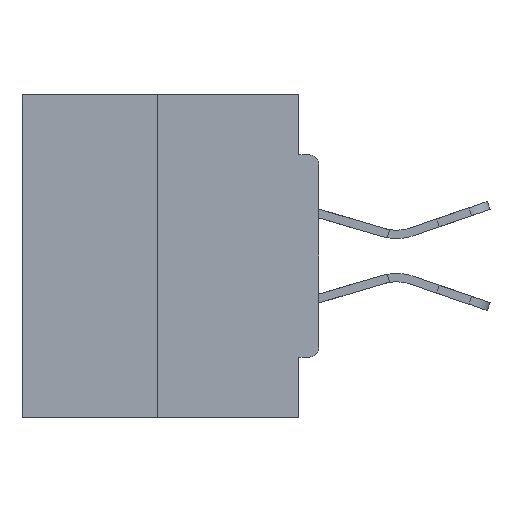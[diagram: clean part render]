
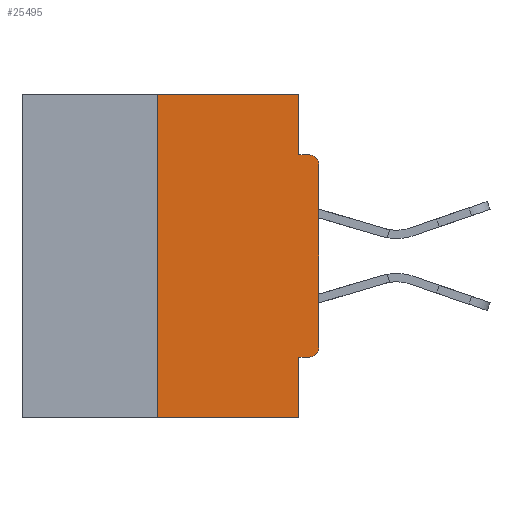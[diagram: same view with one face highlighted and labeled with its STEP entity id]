
A CAD part, left-side view. The second image highlights one B-rep face of the part: STEP entity #25495.
In plain terms, the highlighted planar face has unit normal (-1, 0, 0).
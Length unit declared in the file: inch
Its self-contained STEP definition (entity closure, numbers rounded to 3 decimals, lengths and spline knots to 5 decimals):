
#84 = ORIENTED_EDGE ( 'NONE', *, *, #33081, .F. ) ;
#152 = LINE ( 'NONE', #28186, #579 ) ;
#579 = VECTOR ( 'NONE', #2247, 39.37008 ) ;
#937 = DIRECTION ( 'NONE',  ( 1., 0., 0. ) ) ;
#1289 = VERTEX_POINT ( 'NONE', #6675 ) ;
#1444 = EDGE_CURVE ( 'NONE', #12754, #9517, #26013, .T. ) ;
#2247 = DIRECTION ( 'NONE',  ( 0., -1., 0. ) ) ;
#2290 = DIRECTION ( 'NONE',  ( 0., 0., 1. ) ) ;
#2374 = AXIS2_PLACEMENT_3D ( 'NONE', #28619, #2547, #28486 ) ;
#2547 = DIRECTION ( 'NONE',  ( -1., 0., 0. ) ) ;
#2644 = LINE ( 'NONE', #3035, #33446 ) ;
#3035 = CARTESIAN_POINT ( 'NONE',  ( 0., 0.46, 0. ) ) ;
#3228 = VERTEX_POINT ( 'NONE', #19448 ) ;
#3756 = PLANE ( 'NONE',  #8763 ) ;
#3840 = DIRECTION ( 'NONE',  ( 0., 0., -1. ) ) ;
#4269 = ORIENTED_EDGE ( 'NONE', *, *, #28178, .T. ) ;
#4535 = CARTESIAN_POINT ( 'NONE',  ( 0., 0.031, 0. ) ) ;
#5075 = AXIS2_PLACEMENT_3D ( 'NONE', #9763, #35532, #3840 ) ;
#5079 = EDGE_CURVE ( 'NONE', #5355, #14339, #24553, .T. ) ;
#5355 = VERTEX_POINT ( 'NONE', #33275 ) ;
#6125 = DIRECTION ( 'NONE',  ( 0., 0., -1. ) ) ;
#6675 = CARTESIAN_POINT ( 'NONE',  ( 0., 0.25, 0. ) ) ;
#7234 = EDGE_CURVE ( 'NONE', #9517, #19406, #33463, .T. ) ;
#7672 = EDGE_CURVE ( 'NONE', #36453, #3228, #17174, .T. ) ;
#8690 = CARTESIAN_POINT ( 'NONE',  ( 0., 0., -0.1085 ) ) ;
#8763 = AXIS2_PLACEMENT_3D ( 'NONE', #17320, #937, #26868 ) ;
#9124 = CARTESIAN_POINT ( 'NONE',  ( 0., 0., -0.0935 ) ) ;
#9208 = DIRECTION ( 'NONE',  ( 0., -1., 0. ) ) ;
#9387 = CARTESIAN_POINT ( 'NONE',  ( 0., 0.25, -0.5 ) ) ;
#9517 = VERTEX_POINT ( 'NONE', #10937 ) ;
#9763 = CARTESIAN_POINT ( 'NONE',  ( 0., 0.015, -0.3915 ) ) ;
#10514 = VERTEX_POINT ( 'NONE', #8690 ) ;
#10799 = VECTOR ( 'NONE', #27660, 39.37008 ) ;
#10937 = CARTESIAN_POINT ( 'NONE',  ( 0., 0.031, -0.0935 ) ) ;
#12011 = DIRECTION ( 'NONE',  ( 0., -1., 0. ) ) ;
#12162 = CARTESIAN_POINT ( 'NONE',  ( 0., 0.031, -0.5 ) ) ;
#12621 = LINE ( 'NONE', #24603, #10799 ) ;
#12754 = VERTEX_POINT ( 'NONE', #4535 ) ;
#13917 = CARTESIAN_POINT ( 'NONE',  ( 0., 0., 0. ) ) ;
#14274 = VECTOR ( 'NONE', #15642, 39.37008 ) ;
#14317 = VECTOR ( 'NONE', #25302, 39.37008 ) ;
#14339 = VERTEX_POINT ( 'NONE', #31032 ) ;
#14480 = ORIENTED_EDGE ( 'NONE', *, *, #7234, .F. ) ;
#14607 = ORIENTED_EDGE ( 'NONE', *, *, #34176, .T. ) ;
#15642 = DIRECTION ( 'NONE',  ( 0., 0., -1. ) ) ;
#15994 = CARTESIAN_POINT ( 'NONE',  ( 0., 0.015, -0.4065 ) ) ;
#16292 = ORIENTED_EDGE ( 'NONE', *, *, #23053, .F. ) ;
#17012 = ORIENTED_EDGE ( 'NONE', *, *, #22709, .F. ) ;
#17174 = CIRCLE ( 'NONE', #5075, 0.015 ) ;
#17320 = CARTESIAN_POINT ( 'NONE',  ( 0., 0.46, 0. ) ) ;
#18474 = EDGE_CURVE ( 'NONE', #25018, #14339, #152, .T. ) ;
#19049 = CIRCLE ( 'NONE', #2374, 0.015 ) ;
#19406 = VERTEX_POINT ( 'NONE', #34623 ) ;
#19448 = CARTESIAN_POINT ( 'NONE',  ( 0., 0., -0.3915 ) ) ;
#19876 = CARTESIAN_POINT ( 'NONE',  ( 0., 0.25, 0. ) ) ;
#20106 = LINE ( 'NONE', #13917, #34088 ) ;
#22709 = EDGE_CURVE ( 'NONE', #1289, #12754, #2644, .T. ) ;
#23053 = EDGE_CURVE ( 'NONE', #36453, #5355, #12621, .T. ) ;
#23811 = LINE ( 'NONE', #19876, #14317 ) ;
#24553 = LINE ( 'NONE', #12162, #37203 ) ;
#24603 = CARTESIAN_POINT ( 'NONE',  ( 0., 0., -0.4065 ) ) ;
#24803 = ORIENTED_EDGE ( 'NONE', *, *, #18474, .T. ) ;
#25018 = VERTEX_POINT ( 'NONE', #9387 ) ;
#25302 = DIRECTION ( 'NONE',  ( 0., 0., 1. ) ) ;
#25495 = ADVANCED_FACE ( 'NONE', ( #30035 ), #3756, .F. ) ;
#25791 = VECTOR ( 'NONE', #12011, 39.37008 ) ;
#26013 = LINE ( 'NONE', #36092, #14274 ) ;
#26868 = DIRECTION ( 'NONE',  ( 0., 0., -1. ) ) ;
#27660 = DIRECTION ( 'NONE',  ( 0., 1., 0. ) ) ;
#28178 = EDGE_CURVE ( 'NONE', #3228, #10514, #20106, .T. ) ;
#28186 = CARTESIAN_POINT ( 'NONE',  ( 0., 0.46, -0.5 ) ) ;
#28486 = DIRECTION ( 'NONE',  ( 0., 0., -1. ) ) ;
#28619 = CARTESIAN_POINT ( 'NONE',  ( 0., 0.015, -0.1085 ) ) ;
#29211 = ORIENTED_EDGE ( 'NONE', *, *, #1444, .F. ) ;
#29535 = ORIENTED_EDGE ( 'NONE', *, *, #7672, .T. ) ;
#30035 = FACE_OUTER_BOUND ( 'NONE', #31251, .T. ) ;
#31032 = CARTESIAN_POINT ( 'NONE',  ( 0., 0.031, -0.5 ) ) ;
#31251 = EDGE_LOOP ( 'NONE', ( #17012, #84, #24803, #31597, #16292, #29535, #4269, #14607, #14480, #29211 ) ) ;
#31597 = ORIENTED_EDGE ( 'NONE', *, *, #5079, .F. ) ;
#33081 = EDGE_CURVE ( 'NONE', #25018, #1289, #23811, .T. ) ;
#33275 = CARTESIAN_POINT ( 'NONE',  ( 0., 0.031, -0.4065 ) ) ;
#33446 = VECTOR ( 'NONE', #9208, 39.37008 ) ;
#33463 = LINE ( 'NONE', #9124, #25791 ) ;
#34088 = VECTOR ( 'NONE', #2290, 39.37008 ) ;
#34176 = EDGE_CURVE ( 'NONE', #10514, #19406, #19049, .T. ) ;
#34623 = CARTESIAN_POINT ( 'NONE',  ( 0., 0.015, -0.0935 ) ) ;
#35532 = DIRECTION ( 'NONE',  ( -1., 0., 0. ) ) ;
#36092 = CARTESIAN_POINT ( 'NONE',  ( 0., 0.031, 0. ) ) ;
#36453 = VERTEX_POINT ( 'NONE', #15994 ) ;
#37203 = VECTOR ( 'NONE', #6125, 39.37008 ) ;
